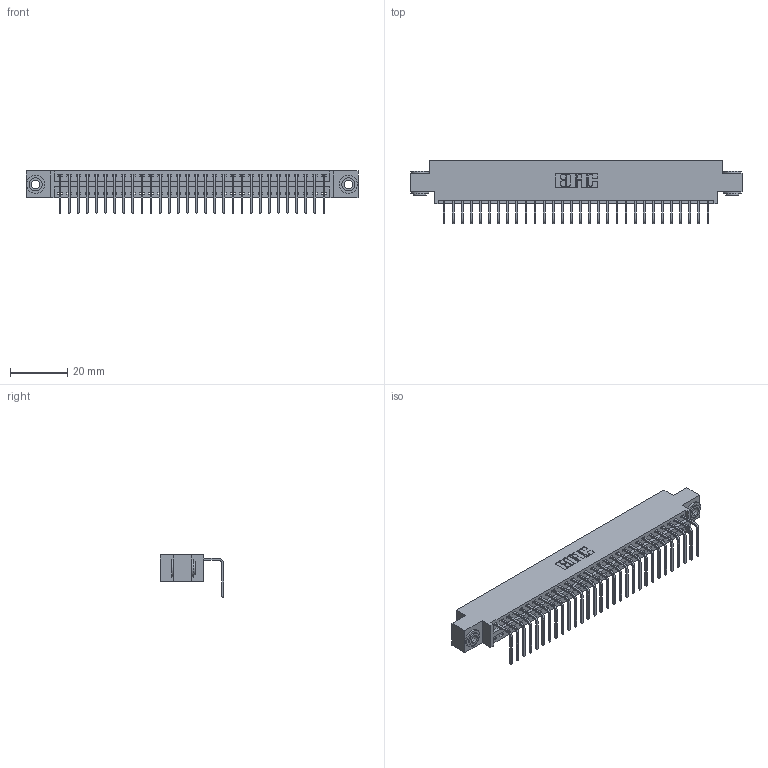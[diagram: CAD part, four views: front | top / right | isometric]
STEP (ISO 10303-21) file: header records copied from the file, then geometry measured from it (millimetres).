
FILE_DESCRIPTION (( 'STEP AP203' ), '1' );
FILE_NAME ('346-030-558-603.STEP', '2022-05-06T16:08:13', ( '' ), ( '' ), 'SwSTEP 2.0', 'SolidWorks 2020', '' );
FILE_SCHEMA (( 'CONFIG_CONTROL_DESIGN' ));
Length unit declared in the file: inch
Products named in the file (4): 346 Part_0.170 Offset - 0.156 Dia-TH; 346-030-558-603; 345-250-002_345-250-002-102; 345-292-001_558 Tail - 2
Assembly tree (33 placements, depth 2):
  346-030-558-603
    346 Part_0.170 Offset - 0.156 Dia-TH
    345-292-001_558 Tail - 2  x30
    345-250-002_345-250-002-102  x2
Bounding box: 115.82 x 22.16 x 14.73 mm (x, y, z)
Volume: 10950.9 mm3; surface area: 14565.8 mm2
Topology: 33 solids, 33 shells, 1978 faces, 5913 edges, 3898 vertices
Faces by surface type: plane 1364, cylinder 606, cone 8
Entity records: 21516 total; most frequent: CARTESIAN_POINT 3675, ORIENTED_EDGE 3630, DIRECTION 3285, EDGE_CURVE 1815, VECTOR 1539, LINE 1539, VERTEX_POINT 1206, AXIS2_PLACEMENT_3D 873
